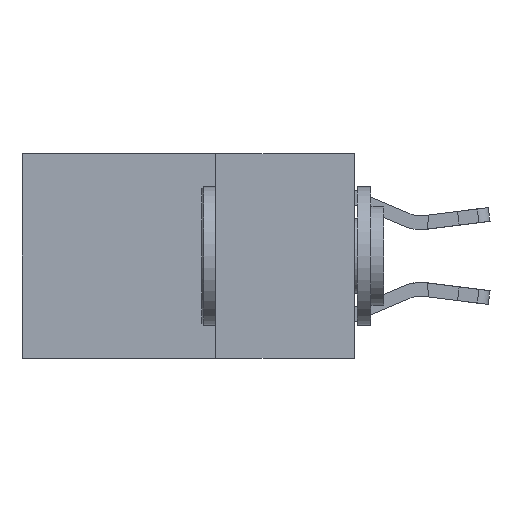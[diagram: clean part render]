
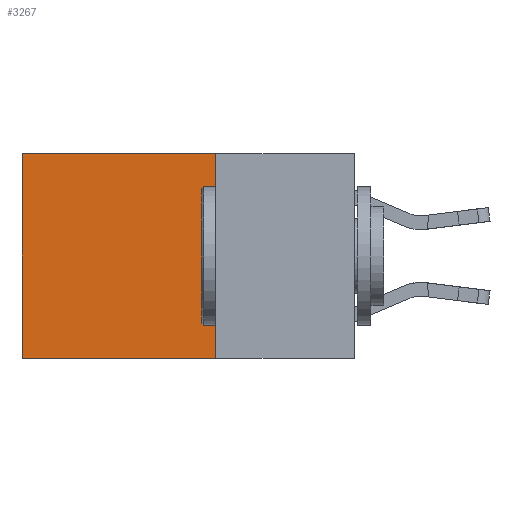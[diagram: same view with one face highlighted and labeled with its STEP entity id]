
A CAD part, left-side view. The second image highlights one B-rep face of the part: STEP entity #3267.
In plain terms, the highlighted planar face has unit normal (-1, 0, 0).
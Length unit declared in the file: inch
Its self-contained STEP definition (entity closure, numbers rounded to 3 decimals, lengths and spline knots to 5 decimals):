
#501 = LINE ( 'NONE', #3005, #5695 ) ;
#1482 = CARTESIAN_POINT ( 'NONE',  ( 0.2625, 0.6, -0.37 ) ) ;
#2284 = LINE ( 'NONE', #17609, #6839 ) ;
#2904 = VERTEX_POINT ( 'NONE', #6342 ) ;
#2998 = VERTEX_POINT ( 'NONE', #24109 ) ;
#3005 = CARTESIAN_POINT ( 'NONE',  ( 0.2625, 0.25, -0.37 ) ) ;
#3267 = ADVANCED_FACE ( 'NONE', ( #14893 ), #26116, .F. ) ;
#3470 = LINE ( 'NONE', #6242, #18782 ) ;
#5285 = EDGE_CURVE ( 'NONE', #2998, #2904, #2284, .T. ) ;
#5591 = ORIENTED_EDGE ( 'NONE', *, *, #7249, .F. ) ;
#5695 = VECTOR ( 'NONE', #24734, 39.37008 ) ;
#6242 = CARTESIAN_POINT ( 'NONE',  ( 0.2625, 0.6, 0. ) ) ;
#6342 = CARTESIAN_POINT ( 'NONE',  ( 0.2625, 0.25, -0.37 ) ) ;
#6666 = DIRECTION ( 'NONE',  ( 0., 1., 0. ) ) ;
#6764 = CARTESIAN_POINT ( 'NONE',  ( 0.2625, 0.6, 0. ) ) ;
#6839 = VECTOR ( 'NONE', #11055, 39.37008 ) ;
#7249 = EDGE_CURVE ( 'NONE', #2904, #28131, #501, .T. ) ;
#8612 = CARTESIAN_POINT ( 'NONE',  ( 0.2625, 0.25, 0. ) ) ;
#9901 = ORIENTED_EDGE ( 'NONE', *, *, #5285, .F. ) ;
#10516 = LINE ( 'NONE', #19400, #18443 ) ;
#11055 = DIRECTION ( 'NONE',  ( 0., 0., -1. ) ) ;
#12378 = EDGE_LOOP ( 'NONE', ( #18026, #5591, #9901, #27083 ) ) ;
#12564 = DIRECTION ( 'NONE',  ( 0., 0., -1. ) ) ;
#12621 = VERTEX_POINT ( 'NONE', #6764 ) ;
#14668 = EDGE_CURVE ( 'NONE', #2998, #12621, #10516, .T. ) ;
#14893 = FACE_OUTER_BOUND ( 'NONE', #12378, .T. ) ;
#17609 = CARTESIAN_POINT ( 'NONE',  ( 0.2625, 0.25, 0. ) ) ;
#18026 = ORIENTED_EDGE ( 'NONE', *, *, #24512, .T. ) ;
#18443 = VECTOR ( 'NONE', #6666, 39.37008 ) ;
#18782 = VECTOR ( 'NONE', #21533, 39.37008 ) ;
#19400 = CARTESIAN_POINT ( 'NONE',  ( 0.2625, 0.25, 0. ) ) ;
#21533 = DIRECTION ( 'NONE',  ( 0., 0., -1. ) ) ;
#21556 = AXIS2_PLACEMENT_3D ( 'NONE', #8612, #23470, #12564 ) ;
#23470 = DIRECTION ( 'NONE',  ( 1., 0., 0. ) ) ;
#24109 = CARTESIAN_POINT ( 'NONE',  ( 0.2625, 0.25, 0. ) ) ;
#24512 = EDGE_CURVE ( 'NONE', #12621, #28131, #3470, .T. ) ;
#24734 = DIRECTION ( 'NONE',  ( 0., 1., 0. ) ) ;
#26116 = PLANE ( 'NONE',  #21556 ) ;
#27083 = ORIENTED_EDGE ( 'NONE', *, *, #14668, .T. ) ;
#28131 = VERTEX_POINT ( 'NONE', #1482 ) ;
